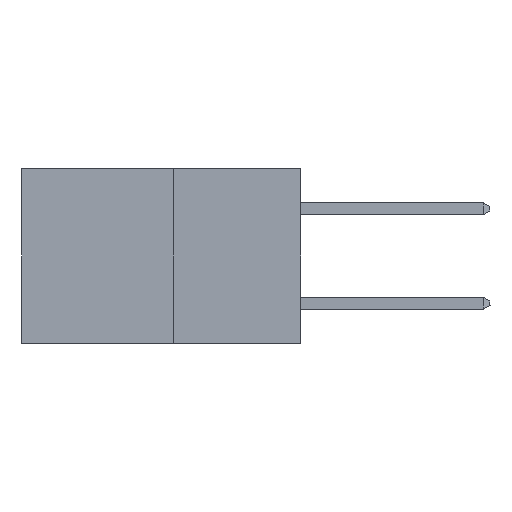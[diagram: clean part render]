
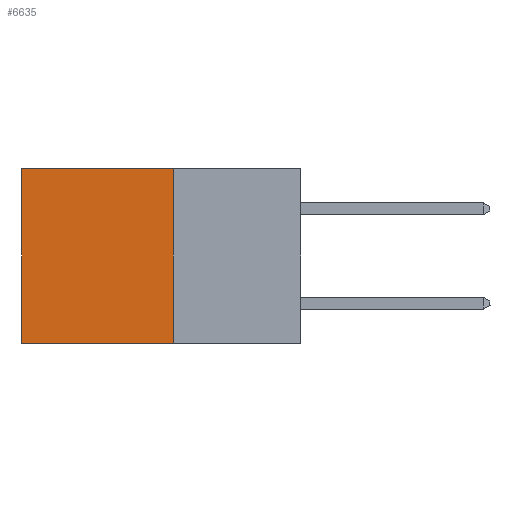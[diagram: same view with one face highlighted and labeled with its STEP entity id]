
A CAD part, left-side view. The second image highlights one B-rep face of the part: STEP entity #6635.
In plain terms, the highlighted planar face has unit normal (-1, 0, 0).
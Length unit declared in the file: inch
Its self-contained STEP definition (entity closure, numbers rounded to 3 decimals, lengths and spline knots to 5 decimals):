
#323 = EDGE_CURVE ( 'NONE', #11053, #7967, #15194, .T. ) ;
#450 = DIRECTION ( 'NONE',  ( 1., 0., 0. ) ) ;
#707 = CARTESIAN_POINT ( 'NONE',  ( 0.277, 0.27, -0.37 ) ) ;
#727 = AXIS2_PLACEMENT_3D ( 'NONE', #17451, #450, #10431 ) ;
#2604 = DIRECTION ( 'NONE',  ( 0., 1., 0. ) ) ;
#3145 = CARTESIAN_POINT ( 'NONE',  ( 0.277, 0.27, 0. ) ) ;
#3686 = EDGE_LOOP ( 'NONE', ( #11856, #14194, #9718, #14324 ) ) ;
#4026 = LINE ( 'NONE', #15985, #15000 ) ;
#4236 = VECTOR ( 'NONE', #9114, 39.37008 ) ;
#5362 = CARTESIAN_POINT ( 'NONE',  ( 0.277, 0.27, 0. ) ) ;
#5522 = FACE_OUTER_BOUND ( 'NONE', #3686, .T. ) ;
#6635 = ADVANCED_FACE ( 'NONE', ( #5522 ), #7514, .F. ) ;
#7274 = CARTESIAN_POINT ( 'NONE',  ( 0.277, 0.59, -0.37 ) ) ;
#7514 = PLANE ( 'NONE',  #727 ) ;
#7519 = VECTOR ( 'NONE', #12106, 39.37008 ) ;
#7711 = CARTESIAN_POINT ( 'NONE',  ( 0.277, 0.27, -0.37 ) ) ;
#7967 = VERTEX_POINT ( 'NONE', #7711 ) ;
#9093 = VECTOR ( 'NONE', #2604, 39.37008 ) ;
#9114 = DIRECTION ( 'NONE',  ( 0., 0., -1. ) ) ;
#9718 = ORIENTED_EDGE ( 'NONE', *, *, #323, .F. ) ;
#9885 = VERTEX_POINT ( 'NONE', #14986 ) ;
#10431 = DIRECTION ( 'NONE',  ( 0., 0., -1. ) ) ;
#10626 = CARTESIAN_POINT ( 'NONE',  ( 0.277, 0.27, -0.37 ) ) ;
#10739 = EDGE_CURVE ( 'NONE', #11053, #9885, #12900, .T. ) ;
#11053 = VERTEX_POINT ( 'NONE', #3145 ) ;
#11356 = LINE ( 'NONE', #707, #7519 ) ;
#11856 = ORIENTED_EDGE ( 'NONE', *, *, #14673, .T. ) ;
#12106 = DIRECTION ( 'NONE',  ( 0., 1., 0. ) ) ;
#12900 = LINE ( 'NONE', #5362, #9093 ) ;
#14194 = ORIENTED_EDGE ( 'NONE', *, *, #16852, .F. ) ;
#14324 = ORIENTED_EDGE ( 'NONE', *, *, #10739, .T. ) ;
#14588 = VERTEX_POINT ( 'NONE', #7274 ) ;
#14673 = EDGE_CURVE ( 'NONE', #9885, #14588, #4026, .T. ) ;
#14986 = CARTESIAN_POINT ( 'NONE',  ( 0.277, 0.59, 0. ) ) ;
#15000 = VECTOR ( 'NONE', #17388, 39.37008 ) ;
#15194 = LINE ( 'NONE', #10626, #4236 ) ;
#15985 = CARTESIAN_POINT ( 'NONE',  ( 0.277, 0.59, -0.37 ) ) ;
#16852 = EDGE_CURVE ( 'NONE', #7967, #14588, #11356, .T. ) ;
#17388 = DIRECTION ( 'NONE',  ( 0., 0., -1. ) ) ;
#17451 = CARTESIAN_POINT ( 'NONE',  ( 0.277, 0.27, -0.37 ) ) ;
